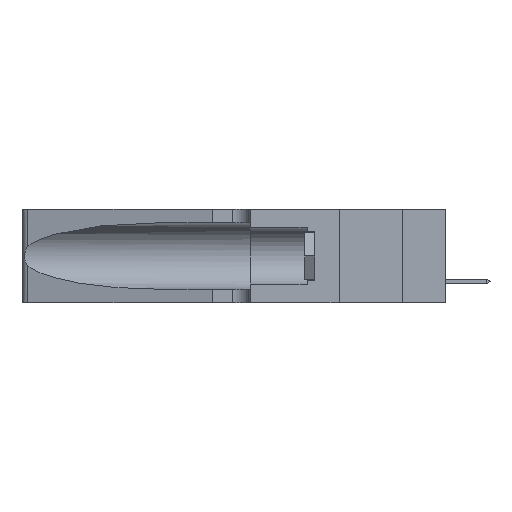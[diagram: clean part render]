
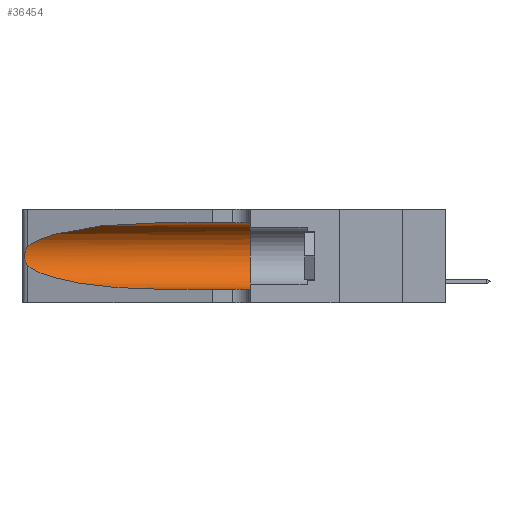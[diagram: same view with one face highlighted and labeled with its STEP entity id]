
A CAD part, left-side view. The second image highlights one B-rep face of the part: STEP entity #36454.
In plain terms, the highlighted cylindrical face has radius 3.308 mm (diameter 6.617 mm), a partial arc.
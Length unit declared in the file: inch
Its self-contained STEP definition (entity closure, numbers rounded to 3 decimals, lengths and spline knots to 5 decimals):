
#352 = VECTOR ( 'NONE', #34938, 39.37008 ) ;
#1153 = CARTESIAN_POINT ( 'NONE',  ( 0.1305, 0.72297, 0.31525 ) ) ;
#1212 = CARTESIAN_POINT ( 'NONE',  ( 0.26075, 1.23896, 0.178 ) ) ;
#2179 = ORIENTED_EDGE ( 'NONE', *, *, #37496, .F. ) ;
#3076 = CIRCLE ( 'NONE', #6266, 0.13025 ) ;
#3457 =( BOUNDED_CURVE ( )  B_SPLINE_CURVE ( 3, ( #38387, #41899, #27032, #15952 ),
 .UNSPECIFIED., .F., .T. ) 
 B_SPLINE_CURVE_WITH_KNOTS ( ( 4, 4 ),
 ( 3.44316, 4.71239 ),
 .UNSPECIFIED. ) 
 CURVE ( )  GEOMETRIC_REPRESENTATION_ITEM ( )  RATIONAL_B_SPLINE_CURVE ( ( 1., 0.87, 0.87, 1. ) ) 
 REPRESENTATION_ITEM ( '' )  );
#3952 = CARTESIAN_POINT ( 'NONE',  ( 0.1305, 0.35, 0.05475 ) ) ;
#4157 = CARTESIAN_POINT ( 'NONE',  ( 0.25555, 1.22994, 0.2215 ) ) ;
#5630 = CARTESIAN_POINT ( 'NONE',  ( 0.1305, 1.61858, 0.31525 ) ) ;
#5975 = CARTESIAN_POINT ( 'NONE',  ( 0.1305, 0.72297, 0.31525 ) ) ;
#6125 = B_SPLINE_CURVE_WITH_KNOTS ( 'NONE', 3,
 ( #37520, #4157, #48106, #19054, #30619, #8172, #19521, #1212, #22946, #23105, #45598, #23267, #27014, #30778 ),
 .UNSPECIFIED., .F., .F.,
 ( 4, 2, 2, 2, 2, 2, 4 ),
 ( 0., 0.00027, 0.00053, 0.00107, 0.0016, 0.00187, 0.00214 ),
 .UNSPECIFIED. ) ;
#6266 = AXIS2_PLACEMENT_3D ( 'NONE', #7563, #15022, #26243 ) ;
#6467 = ORIENTED_EDGE ( 'NONE', *, *, #42172, .F. ) ;
#7563 = CARTESIAN_POINT ( 'NONE',  ( 0.1305, 0.35, 0.185 ) ) ;
#8172 = CARTESIAN_POINT ( 'NONE',  ( 0.26018, 1.23835, 0.19895 ) ) ;
#9670 = VERTEX_POINT ( 'NONE', #46674 ) ;
#10270 = LINE ( 'NONE', #5630, #352 ) ;
#12648 = CARTESIAN_POINT ( 'NONE',  ( 0.2373, 1.15595, 0.28018 ) ) ;
#13975 = ORIENTED_EDGE ( 'NONE', *, *, #28698, .T. ) ;
#15022 = DIRECTION ( 'NONE',  ( 0., 1., 0. ) ) ;
#15952 = CARTESIAN_POINT ( 'NONE',  ( 0.1305, 0.72297, 0.05475 ) ) ;
#17445 = VECTOR ( 'NONE', #38225, 39.37008 ) ;
#19054 = CARTESIAN_POINT ( 'NONE',  ( 0.25787, 1.23484, 0.2124 ) ) ;
#19521 = CARTESIAN_POINT ( 'NONE',  ( 0.26075, 1.23896, 0.19203 ) ) ;
#19872 = VERTEX_POINT ( 'NONE', #35296 ) ;
#21753 = DIRECTION ( 'NONE',  ( 0., 0., -1. ) ) ;
#22946 = CARTESIAN_POINT ( 'NONE',  ( 0.26017, 1.23833, 0.17102 ) ) ;
#23105 = CARTESIAN_POINT ( 'NONE',  ( 0.25856, 1.23593, 0.16098 ) ) ;
#23267 = CARTESIAN_POINT ( 'NONE',  ( 0.25639, 1.23186, 0.15144 ) ) ;
#23702 = CARTESIAN_POINT ( 'NONE',  ( 0.25487, 1.22718, 0.22369 ) ) ;
#24264 = EDGE_CURVE ( 'NONE', #34969, #9670, #40176, .T. ) ;
#24906 = AXIS2_PLACEMENT_3D ( 'NONE', #43935, #29401, #21753 ) ;
#26243 = DIRECTION ( 'NONE',  ( 0., 0., 1. ) ) ;
#27014 = CARTESIAN_POINT ( 'NONE',  ( 0.25555, 1.22993, 0.14849 ) ) ;
#27032 = CARTESIAN_POINT ( 'NONE',  ( 0.18966, 0.96281, 0.05475 ) ) ;
#27546 = FACE_OUTER_BOUND ( 'NONE', #35014, .T. ) ;
#28698 = EDGE_CURVE ( 'NONE', #34745, #34207, #47185, .T. ) ;
#29401 = DIRECTION ( 'NONE',  ( 0., -1., 0. ) ) ;
#29623 = EDGE_CURVE ( 'NONE', #9670, #31026, #6125, .T. ) ;
#30619 = CARTESIAN_POINT ( 'NONE',  ( 0.25854, 1.2359, 0.20912 ) ) ;
#30778 = CARTESIAN_POINT ( 'NONE',  ( 0.25487, 1.22718, 0.14631 ) ) ;
#31026 = VERTEX_POINT ( 'NONE', #37002 ) ;
#32441 = ORIENTED_EDGE ( 'NONE', *, *, #33701, .T. ) ;
#32570 = ORIENTED_EDGE ( 'NONE', *, *, #29623, .T. ) ;
#33701 = EDGE_CURVE ( 'NONE', #31026, #34745, #3457, .T. ) ;
#34207 = VERTEX_POINT ( 'NONE', #3952 ) ;
#34745 = VERTEX_POINT ( 'NONE', #42574 ) ;
#34827 = CARTESIAN_POINT ( 'NONE',  ( 0.18966, 0.96281, 0.31525 ) ) ;
#34938 = DIRECTION ( 'NONE',  ( 0., -1., 0. ) ) ;
#34959 = CARTESIAN_POINT ( 'NONE',  ( 0.1305, 1.61858, 0.05475 ) ) ;
#34969 = VERTEX_POINT ( 'NONE', #5975 ) ;
#35014 = EDGE_LOOP ( 'NONE', ( #46428, #32570, #32441, #13975, #2179, #6467 ) ) ;
#35296 = CARTESIAN_POINT ( 'NONE',  ( 0.1305, 0.35, 0.31525 ) ) ;
#36454 = ADVANCED_FACE ( 'NONE', ( #27546 ), #46823, .F. ) ;
#37002 = CARTESIAN_POINT ( 'NONE',  ( 0.25487, 1.22718, 0.14631 ) ) ;
#37496 = EDGE_CURVE ( 'NONE', #19872, #34207, #3076, .T. ) ;
#37520 = CARTESIAN_POINT ( 'NONE',  ( 0.25487, 1.22718, 0.22369 ) ) ;
#38225 = DIRECTION ( 'NONE',  ( 0., -1., 0. ) ) ;
#38387 = CARTESIAN_POINT ( 'NONE',  ( 0.25487, 1.22718, 0.14631 ) ) ;
#40176 =( BOUNDED_CURVE ( )  B_SPLINE_CURVE ( 3, ( #1153, #34827, #12648, #23702 ),
 .UNSPECIFIED., .F., .F. ) 
 B_SPLINE_CURVE_WITH_KNOTS ( ( 4, 4 ),
 ( 1.5708, 2.84003 ),
 .UNSPECIFIED. ) 
 CURVE ( )  GEOMETRIC_REPRESENTATION_ITEM ( )  RATIONAL_B_SPLINE_CURVE ( ( 1., 0.87, 0.87, 1. ) ) 
 REPRESENTATION_ITEM ( '' )  );
#41899 = CARTESIAN_POINT ( 'NONE',  ( 0.2373, 1.15595, 0.08982 ) ) ;
#42172 = EDGE_CURVE ( 'NONE', #34969, #19872, #10270, .T. ) ;
#42574 = CARTESIAN_POINT ( 'NONE',  ( 0.1305, 0.72297, 0.05475 ) ) ;
#43935 = CARTESIAN_POINT ( 'NONE',  ( 0.1305, 1.61858, 0.185 ) ) ;
#45598 = CARTESIAN_POINT ( 'NONE',  ( 0.25789, 1.23486, 0.15765 ) ) ;
#46428 = ORIENTED_EDGE ( 'NONE', *, *, #24264, .T. ) ;
#46674 = CARTESIAN_POINT ( 'NONE',  ( 0.25487, 1.22718, 0.22369 ) ) ;
#46823 = CYLINDRICAL_SURFACE ( 'NONE', #24906, 0.13025 ) ;
#47185 = LINE ( 'NONE', #34959, #17445 ) ;
#48106 = CARTESIAN_POINT ( 'NONE',  ( 0.25639, 1.23184, 0.21858 ) ) ;
